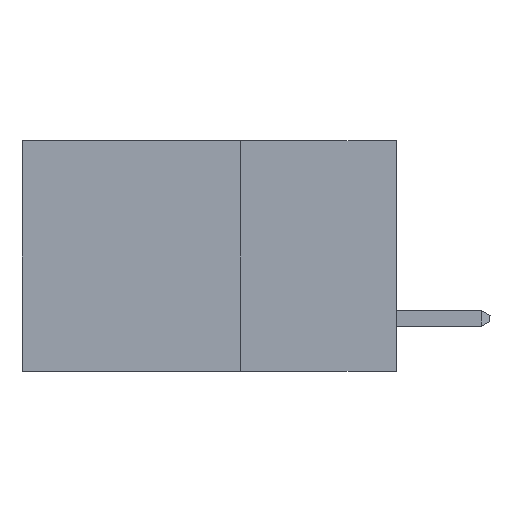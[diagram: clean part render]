
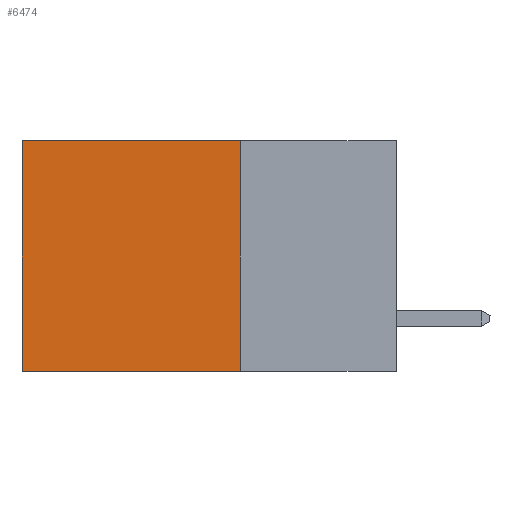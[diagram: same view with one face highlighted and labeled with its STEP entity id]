
A CAD part, left-side view. The second image highlights one B-rep face of the part: STEP entity #6474.
In plain terms, the highlighted planar face has unit normal (-1, 0, 0).
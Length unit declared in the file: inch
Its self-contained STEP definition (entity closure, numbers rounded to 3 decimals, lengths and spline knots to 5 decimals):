
#78 = CARTESIAN_POINT ( 'NONE',  ( 0.2615, 0.25, -0.37 ) ) ;
#1109 = DIRECTION ( 'NONE',  ( 0., 0., -1. ) ) ;
#2628 = EDGE_CURVE ( 'NONE', #6316, #3127, #10884, .T. ) ;
#2805 = EDGE_CURVE ( 'NONE', #5619, #5388, #5397, .T. ) ;
#3127 = VERTEX_POINT ( 'NONE', #8451 ) ;
#3558 = DIRECTION ( 'NONE',  ( 0., 1., 0. ) ) ;
#3783 = CARTESIAN_POINT ( 'NONE',  ( 0.2615, 0.6, 0. ) ) ;
#5388 = VERTEX_POINT ( 'NONE', #16535 ) ;
#5397 = LINE ( 'NONE', #14768, #18415 ) ;
#5619 = VERTEX_POINT ( 'NONE', #3783 ) ;
#5688 = DIRECTION ( 'NONE',  ( 1., 0., 0. ) ) ;
#5771 = EDGE_LOOP ( 'NONE', ( #17917, #11191, #17939, #13255 ) ) ;
#6024 = VECTOR ( 'NONE', #3558, 39.37008 ) ;
#6160 = DIRECTION ( 'NONE',  ( 0., 1., 0. ) ) ;
#6316 = VERTEX_POINT ( 'NONE', #8097 ) ;
#6474 = ADVANCED_FACE ( 'NONE', ( #13273 ), #16161, .F. ) ;
#7095 = DIRECTION ( 'NONE',  ( 0., 0., -1. ) ) ;
#7788 = CARTESIAN_POINT ( 'NONE',  ( 0.2615, 0.25, -0.37 ) ) ;
#7902 = VECTOR ( 'NONE', #8186, 39.37008 ) ;
#8097 = CARTESIAN_POINT ( 'NONE',  ( 0.2615, 0.25, 0. ) ) ;
#8186 = DIRECTION ( 'NONE',  ( 0., 0., -1. ) ) ;
#8451 = CARTESIAN_POINT ( 'NONE',  ( 0.2615, 0.25, -0.37 ) ) ;
#10884 = LINE ( 'NONE', #7788, #7902 ) ;
#11191 = ORIENTED_EDGE ( 'NONE', *, *, #17484, .F. ) ;
#13255 = ORIENTED_EDGE ( 'NONE', *, *, #19223, .T. ) ;
#13273 = FACE_OUTER_BOUND ( 'NONE', #5771, .T. ) ;
#13724 = LINE ( 'NONE', #78, #19645 ) ;
#13924 = LINE ( 'NONE', #14604, #6024 ) ;
#14604 = CARTESIAN_POINT ( 'NONE',  ( 0.2615, 0.25, 0. ) ) ;
#14768 = CARTESIAN_POINT ( 'NONE',  ( 0.2615, 0.6, -0.37 ) ) ;
#16161 = PLANE ( 'NONE',  #17654 ) ;
#16535 = CARTESIAN_POINT ( 'NONE',  ( 0.2615, 0.6, -0.37 ) ) ;
#17484 = EDGE_CURVE ( 'NONE', #3127, #5388, #13724, .T. ) ;
#17539 = CARTESIAN_POINT ( 'NONE',  ( 0.2615, 0.25, -0.37 ) ) ;
#17654 = AXIS2_PLACEMENT_3D ( 'NONE', #17539, #5688, #7095 ) ;
#17917 = ORIENTED_EDGE ( 'NONE', *, *, #2805, .T. ) ;
#17939 = ORIENTED_EDGE ( 'NONE', *, *, #2628, .F. ) ;
#18415 = VECTOR ( 'NONE', #1109, 39.37008 ) ;
#19223 = EDGE_CURVE ( 'NONE', #6316, #5619, #13924, .T. ) ;
#19645 = VECTOR ( 'NONE', #6160, 39.37008 ) ;
